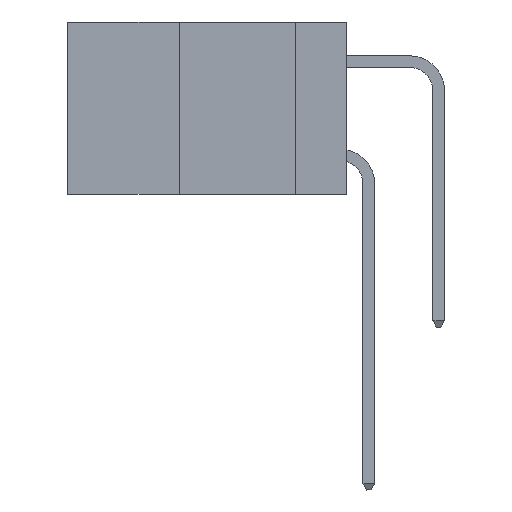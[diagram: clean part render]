
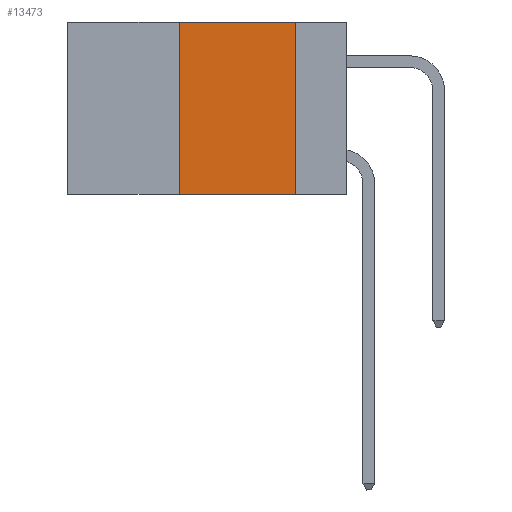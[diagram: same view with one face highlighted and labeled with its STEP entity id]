
A CAD part, left-side view. The second image highlights one B-rep face of the part: STEP entity #13473.
In plain terms, the highlighted planar face has unit normal (-1, 0, 0).
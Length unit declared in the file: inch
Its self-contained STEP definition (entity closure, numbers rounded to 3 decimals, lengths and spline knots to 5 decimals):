
#468 = VERTEX_POINT ( 'NONE', #6438 ) ;
#1185 = VECTOR ( 'NONE', #16456, 39.37008 ) ;
#1211 = ORIENTED_EDGE ( 'NONE', *, *, #15908, .F. ) ;
#1657 = CARTESIAN_POINT ( 'NONE',  ( 0., 0.36, 0. ) ) ;
#1820 = VECTOR ( 'NONE', #16234, 39.37008 ) ;
#2267 = AXIS2_PLACEMENT_3D ( 'NONE', #14353, #5170, #9477 ) ;
#2975 = DIRECTION ( 'NONE',  ( 0., 0., 1. ) ) ;
#3501 = ORIENTED_EDGE ( 'NONE', *, *, #8671, .F. ) ;
#4689 = EDGE_CURVE ( 'NONE', #13368, #6138, #8204, .T. ) ;
#5170 = DIRECTION ( 'NONE',  ( 1., 0., 0. ) ) ;
#5351 = ORIENTED_EDGE ( 'NONE', *, *, #15907, .F. ) ;
#5954 = CARTESIAN_POINT ( 'NONE',  ( 0., 0.11, 0. ) ) ;
#6138 = VERTEX_POINT ( 'NONE', #9507 ) ;
#6438 = CARTESIAN_POINT ( 'NONE',  ( 0., 0.36, 0. ) ) ;
#6854 = FACE_OUTER_BOUND ( 'NONE', #13498, .T. ) ;
#8204 = LINE ( 'NONE', #8298, #1820 ) ;
#8298 = CARTESIAN_POINT ( 'NONE',  ( 0., 0.6, -0.37 ) ) ;
#8671 = EDGE_CURVE ( 'NONE', #12892, #6138, #13975, .T. ) ;
#9015 = LINE ( 'NONE', #1657, #12095 ) ;
#9477 = DIRECTION ( 'NONE',  ( 0., 0., -1. ) ) ;
#9507 = CARTESIAN_POINT ( 'NONE',  ( 0., 0.11, -0.37 ) ) ;
#9671 = DIRECTION ( 'NONE',  ( 0., -1., 0. ) ) ;
#9912 = CARTESIAN_POINT ( 'NONE',  ( 0., 0.11, 0. ) ) ;
#10465 = PLANE ( 'NONE',  #2267 ) ;
#10920 = CARTESIAN_POINT ( 'NONE',  ( 0., 0.6, 0. ) ) ;
#12095 = VECTOR ( 'NONE', #2975, 39.37008 ) ;
#12517 = CARTESIAN_POINT ( 'NONE',  ( 0., 0.36, -0.37 ) ) ;
#12892 = VERTEX_POINT ( 'NONE', #5954 ) ;
#13368 = VERTEX_POINT ( 'NONE', #12517 ) ;
#13473 = ADVANCED_FACE ( 'NONE', ( #6854 ), #10465, .F. ) ;
#13498 = EDGE_LOOP ( 'NONE', ( #3501, #5351, #1211, #16076 ) ) ;
#13975 = LINE ( 'NONE', #9912, #1185 ) ;
#14353 = CARTESIAN_POINT ( 'NONE',  ( 0., 0.6, 0. ) ) ;
#15424 = VECTOR ( 'NONE', #9671, 39.37008 ) ;
#15907 = EDGE_CURVE ( 'NONE', #468, #12892, #16658, .T. ) ;
#15908 = EDGE_CURVE ( 'NONE', #13368, #468, #9015, .T. ) ;
#16076 = ORIENTED_EDGE ( 'NONE', *, *, #4689, .T. ) ;
#16234 = DIRECTION ( 'NONE',  ( 0., -1., 0. ) ) ;
#16456 = DIRECTION ( 'NONE',  ( 0., 0., -1. ) ) ;
#16658 = LINE ( 'NONE', #10920, #15424 ) ;
